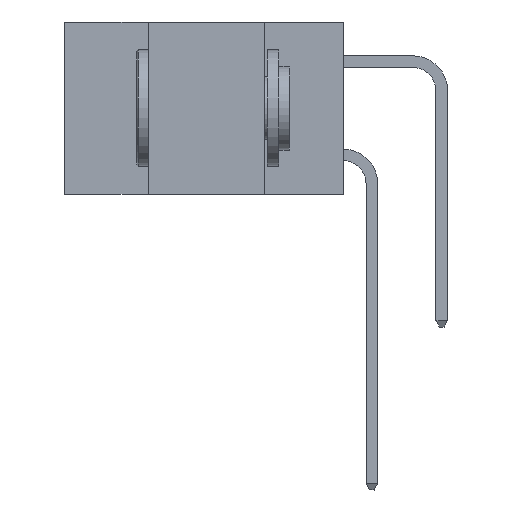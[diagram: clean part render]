
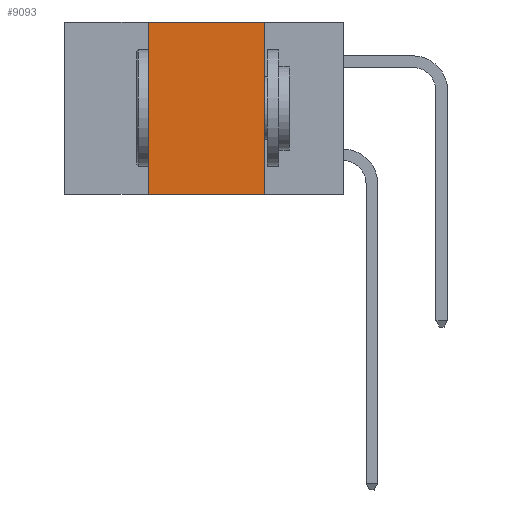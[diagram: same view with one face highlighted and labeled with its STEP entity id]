
A CAD part, left-side view. The second image highlights one B-rep face of the part: STEP entity #9093.
In plain terms, the highlighted planar face has unit normal (-1, 0, 0).
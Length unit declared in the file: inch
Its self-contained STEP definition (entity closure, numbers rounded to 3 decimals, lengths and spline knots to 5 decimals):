
#108 = VECTOR ( 'NONE', #2304, 39.37008 ) ;
#259 = CARTESIAN_POINT ( 'NONE',  ( 0., 0.42, 0. ) ) ;
#389 = CARTESIAN_POINT ( 'NONE',  ( 0., 0.17, 0. ) ) ;
#486 = ORIENTED_EDGE ( 'NONE', *, *, #4660, .F. ) ;
#1761 = VERTEX_POINT ( 'NONE', #17932 ) ;
#2304 = DIRECTION ( 'NONE',  ( 0., -1., 0. ) ) ;
#2674 = DIRECTION ( 'NONE',  ( 0., 0., -1. ) ) ;
#2742 = LINE ( 'NONE', #9391, #108 ) ;
#3133 = DIRECTION ( 'NONE',  ( 0., 0., 1. ) ) ;
#4513 = EDGE_CURVE ( 'NONE', #12610, #8017, #17563, .T. ) ;
#4660 = EDGE_CURVE ( 'NONE', #5524, #12610, #9787, .T. ) ;
#5524 = VERTEX_POINT ( 'NONE', #7779 ) ;
#5748 = EDGE_LOOP ( 'NONE', ( #11829, #486, #17849, #13901 ) ) ;
#6622 = DIRECTION ( 'NONE',  ( 0., 0., -1. ) ) ;
#7779 = CARTESIAN_POINT ( 'NONE',  ( 0., 0.42, 0. ) ) ;
#8017 = VERTEX_POINT ( 'NONE', #13212 ) ;
#8054 = DIRECTION ( 'NONE',  ( 1., 0., 0. ) ) ;
#8726 = EDGE_CURVE ( 'NONE', #1761, #8017, #2742, .T. ) ;
#8970 = EDGE_CURVE ( 'NONE', #1761, #5524, #13827, .T. ) ;
#9002 = DIRECTION ( 'NONE',  ( 0., -1., 0. ) ) ;
#9093 = ADVANCED_FACE ( 'NONE', ( #14755 ), #15189, .F. ) ;
#9391 = CARTESIAN_POINT ( 'NONE',  ( 0., 0.6, -0.37 ) ) ;
#9787 = LINE ( 'NONE', #11423, #17977 ) ;
#11345 = CARTESIAN_POINT ( 'NONE',  ( 0., 0.17, 0. ) ) ;
#11423 = CARTESIAN_POINT ( 'NONE',  ( 0., 0.6, 0. ) ) ;
#11829 = ORIENTED_EDGE ( 'NONE', *, *, #4513, .F. ) ;
#12610 = VERTEX_POINT ( 'NONE', #11345 ) ;
#13212 = CARTESIAN_POINT ( 'NONE',  ( 0., 0.17, -0.37 ) ) ;
#13753 = CARTESIAN_POINT ( 'NONE',  ( 0., 0.6, 0. ) ) ;
#13781 = VECTOR ( 'NONE', #2674, 39.37008 ) ;
#13827 = LINE ( 'NONE', #259, #14290 ) ;
#13901 = ORIENTED_EDGE ( 'NONE', *, *, #8726, .T. ) ;
#14290 = VECTOR ( 'NONE', #3133, 39.37008 ) ;
#14755 = FACE_OUTER_BOUND ( 'NONE', #5748, .T. ) ;
#15152 = AXIS2_PLACEMENT_3D ( 'NONE', #13753, #8054, #6622 ) ;
#15189 = PLANE ( 'NONE',  #15152 ) ;
#17563 = LINE ( 'NONE', #389, #13781 ) ;
#17849 = ORIENTED_EDGE ( 'NONE', *, *, #8970, .F. ) ;
#17932 = CARTESIAN_POINT ( 'NONE',  ( 0., 0.42, -0.37 ) ) ;
#17977 = VECTOR ( 'NONE', #9002, 39.37008 ) ;
